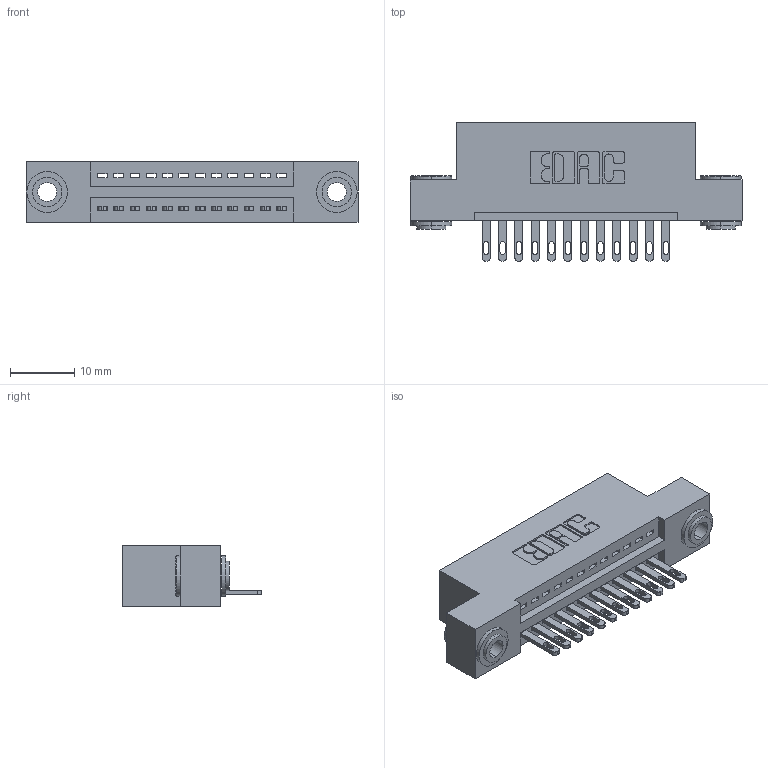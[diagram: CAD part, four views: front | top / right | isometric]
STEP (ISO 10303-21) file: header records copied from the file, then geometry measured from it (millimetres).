
FILE_DESCRIPTION (( 'STEP AP203' ), '1' );
FILE_NAME ('895-012-500-103.STEP', '2020-09-25T01:08:06', ( '' ), ( '' ), 'SwSTEP 2.0', 'SolidWorks 2020', '' );
FILE_SCHEMA (( 'CONFIG_CONTROL_DESIGN' ));
Length unit declared in the file: inch
Products named in the file (4): 345-250-002_345-250-002-102; 345-292-001_345-293-100; 895-012-500-103; 845 Part_Flush Mounting Lugs - 0.156 Dia-TH
Assembly tree (15 placements, depth 2):
  895-012-500-103
    845 Part_Flush Mounting Lugs - 0.156 Dia-TH
    345-292-001_345-293-100  x12
    345-250-002_345-250-002-102  x2
Bounding box: 51.69 x 21.51 x 9.4 mm (x, y, z)
Volume: 4690.5 mm3; surface area: 6067 mm2
Topology: 15 solids, 15 shells, 812 faces, 2433 edges, 1618 vertices
Faces by surface type: plane 498, cylinder 306, cone 8
Entity records: 13650 total; most frequent: CARTESIAN_POINT 2343, ORIENTED_EDGE 2282, DIRECTION 2123, EDGE_CURVE 1141, LINE 933, VECTOR 933, VERTEX_POINT 758, AXIS2_PLACEMENT_3D 595
